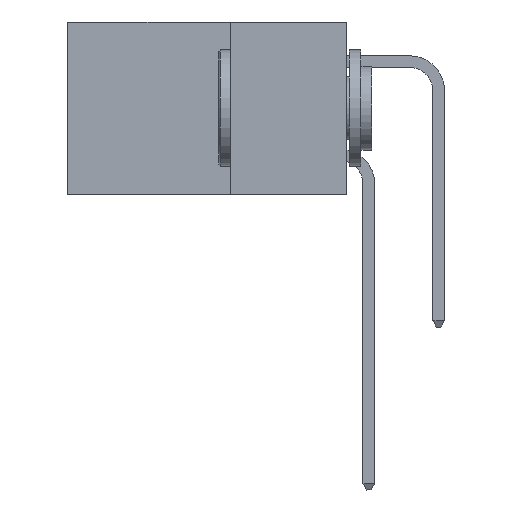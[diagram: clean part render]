
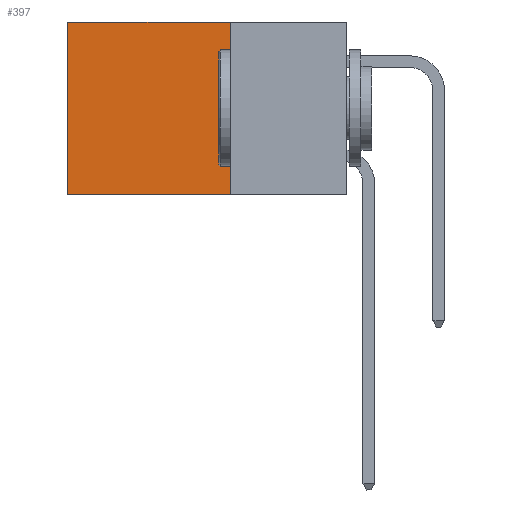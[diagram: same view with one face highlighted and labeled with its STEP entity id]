
A CAD part, left-side view. The second image highlights one B-rep face of the part: STEP entity #397.
In plain terms, the highlighted planar face has unit normal (-1, 0, 0).
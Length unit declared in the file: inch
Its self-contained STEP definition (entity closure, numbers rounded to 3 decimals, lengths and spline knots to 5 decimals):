
#107 = VECTOR ( 'NONE', #11948, 39.37008 ) ;
#238 = CARTESIAN_POINT ( 'NONE',  ( 0.2875, 0.25, 0. ) ) ;
#397 = ADVANCED_FACE ( 'NONE', ( #10609 ), #4282, .F. ) ;
#960 = CARTESIAN_POINT ( 'NONE',  ( 0.2875, 0.6, 0. ) ) ;
#1717 = ORIENTED_EDGE ( 'NONE', *, *, #12882, .T. ) ;
#1991 = LINE ( 'NONE', #12886, #14061 ) ;
#2359 = ORIENTED_EDGE ( 'NONE', *, *, #2406, .T. ) ;
#2406 = EDGE_CURVE ( 'NONE', #2554, #9350, #10168, .T. ) ;
#2431 = EDGE_LOOP ( 'NONE', ( #1717, #4205, #11807, #2359 ) ) ;
#2554 = VERTEX_POINT ( 'NONE', #2951 ) ;
#2951 = CARTESIAN_POINT ( 'NONE',  ( 0.2875, 0.25, 0. ) ) ;
#3526 = EDGE_CURVE ( 'NONE', #2554, #7699, #11070, .T. ) ;
#3738 = VERTEX_POINT ( 'NONE', #10655 ) ;
#3846 = CARTESIAN_POINT ( 'NONE',  ( 0.2875, 0.25, -0.37 ) ) ;
#3914 = VECTOR ( 'NONE', #12724, 39.37008 ) ;
#4205 = ORIENTED_EDGE ( 'NONE', *, *, #14949, .F. ) ;
#4252 = DIRECTION ( 'NONE',  ( 1., 0., 0. ) ) ;
#4282 = PLANE ( 'NONE',  #6118 ) ;
#6118 = AXIS2_PLACEMENT_3D ( 'NONE', #15660, #4252, #15719 ) ;
#6782 = LINE ( 'NONE', #960, #107 ) ;
#6956 = VECTOR ( 'NONE', #15196, 39.37008 ) ;
#7699 = VERTEX_POINT ( 'NONE', #3846 ) ;
#9350 = VERTEX_POINT ( 'NONE', #14235 ) ;
#10168 = LINE ( 'NONE', #238, #6956 ) ;
#10609 = FACE_OUTER_BOUND ( 'NONE', #2431, .T. ) ;
#10655 = CARTESIAN_POINT ( 'NONE',  ( 0.2875, 0.6, -0.37 ) ) ;
#11070 = LINE ( 'NONE', #12933, #3914 ) ;
#11807 = ORIENTED_EDGE ( 'NONE', *, *, #3526, .F. ) ;
#11948 = DIRECTION ( 'NONE',  ( 0., 0., -1. ) ) ;
#12724 = DIRECTION ( 'NONE',  ( 0., 0., -1. ) ) ;
#12882 = EDGE_CURVE ( 'NONE', #9350, #3738, #6782, .T. ) ;
#12886 = CARTESIAN_POINT ( 'NONE',  ( 0.2875, 0.25, -0.37 ) ) ;
#12933 = CARTESIAN_POINT ( 'NONE',  ( 0.2875, 0.25, 0. ) ) ;
#14061 = VECTOR ( 'NONE', #14123, 39.37008 ) ;
#14123 = DIRECTION ( 'NONE',  ( 0., 1., 0. ) ) ;
#14235 = CARTESIAN_POINT ( 'NONE',  ( 0.2875, 0.6, 0. ) ) ;
#14949 = EDGE_CURVE ( 'NONE', #7699, #3738, #1991, .T. ) ;
#15196 = DIRECTION ( 'NONE',  ( 0., 1., 0. ) ) ;
#15660 = CARTESIAN_POINT ( 'NONE',  ( 0.2875, 0.25, 0. ) ) ;
#15719 = DIRECTION ( 'NONE',  ( 0., 0., -1. ) ) ;
